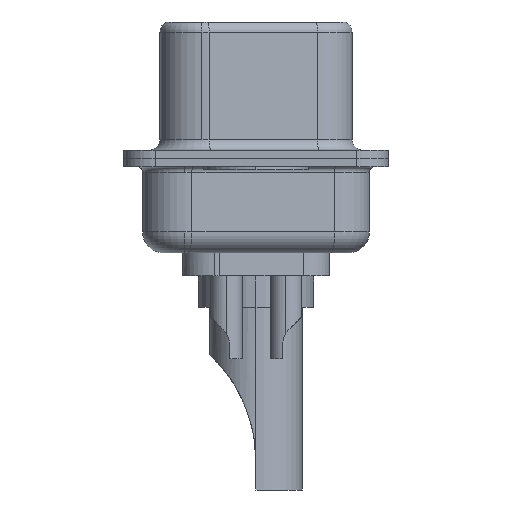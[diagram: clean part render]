
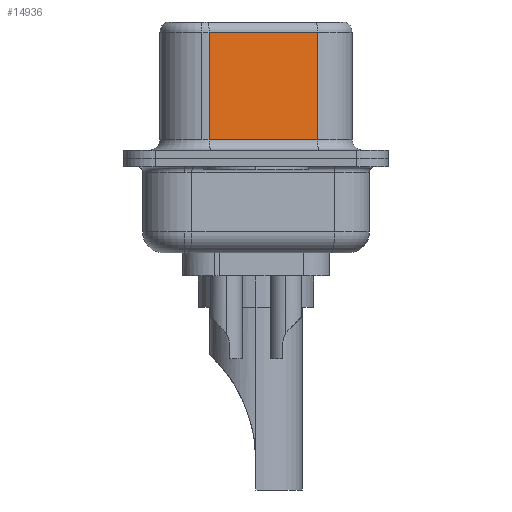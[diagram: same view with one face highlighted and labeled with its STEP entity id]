
A CAD part, left-side view. The second image highlights one B-rep face of the part: STEP entity #14936.
In plain terms, the highlighted planar face has unit normal (-0.985, -0.174, 0).
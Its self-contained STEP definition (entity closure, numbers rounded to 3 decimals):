
#769 = ORIENTED_EDGE ( 'NONE', *, *, #3355, .T. ) ;
#988 = DIRECTION ( 'NONE',  ( 0., 0., -1. ) ) ;
#1220 = VECTOR ( 'NONE', #13043, 1000. ) ;
#1666 = EDGE_CURVE ( 'NONE', #3581, #12307, #10937, .T. ) ;
#2328 = VECTOR ( 'NONE', #5864, 1000. ) ;
#3355 = EDGE_CURVE ( 'NONE', #6122, #3581, #7586, .T. ) ;
#3581 = VERTEX_POINT ( 'NONE', #12643 ) ;
#3767 = AXIS2_PLACEMENT_3D ( 'NONE', #15547, #12094, #4755 ) ;
#4089 = DIRECTION ( 'NONE',  ( 0., 0., -1. ) ) ;
#4755 = DIRECTION ( 'NONE',  ( -0.174, 0.985, 0. ) ) ;
#5244 = EDGE_LOOP ( 'NONE', ( #8255, #769, #15324, #13079 ) ) ;
#5864 = DIRECTION ( 'NONE',  ( 0.174, -0.985, 0. ) ) ;
#6122 = VERTEX_POINT ( 'NONE', #8403 ) ;
#6999 = FACE_OUTER_BOUND ( 'NONE', #5244, .T. ) ;
#7586 = LINE ( 'NONE', #11459, #1220 ) ;
#8171 = CARTESIAN_POINT ( 'NONE',  ( 4.565, -2.927, 6.52 ) ) ;
#8255 = ORIENTED_EDGE ( 'NONE', *, *, #9548, .F. ) ;
#8403 = CARTESIAN_POINT ( 'NONE',  ( 4.565, -2.927, 6.02 ) ) ;
#8763 = CARTESIAN_POINT ( 'NONE',  ( 3.655, 2.233, 6.52 ) ) ;
#9102 = VECTOR ( 'NONE', #988, 1000. ) ;
#9497 = LINE ( 'NONE', #8171, #9102 ) ;
#9548 = EDGE_CURVE ( 'NONE', #6122, #14612, #9497, .T. ) ;
#9572 = EDGE_CURVE ( 'NONE', #12307, #14612, #15115, .T. ) ;
#9593 = PLANE ( 'NONE',  #3767 ) ;
#10266 = CARTESIAN_POINT ( 'NONE',  ( 4.565, -2.927, 0.9 ) ) ;
#10937 = LINE ( 'NONE', #8763, #13698 ) ;
#11459 = CARTESIAN_POINT ( 'NONE',  ( 4.565, -2.927, 6.02 ) ) ;
#11978 = CARTESIAN_POINT ( 'NONE',  ( 4.565, -2.927, 0.9 ) ) ;
#12094 = DIRECTION ( 'NONE',  ( 0.985, 0.174, 0. ) ) ;
#12307 = VERTEX_POINT ( 'NONE', #14799 ) ;
#12643 = CARTESIAN_POINT ( 'NONE',  ( 3.655, 2.233, 6.02 ) ) ;
#13043 = DIRECTION ( 'NONE',  ( -0.174, 0.985, 0. ) ) ;
#13079 = ORIENTED_EDGE ( 'NONE', *, *, #9572, .T. ) ;
#13698 = VECTOR ( 'NONE', #4089, 1000. ) ;
#14612 = VERTEX_POINT ( 'NONE', #10266 ) ;
#14799 = CARTESIAN_POINT ( 'NONE',  ( 3.655, 2.233, 0.9 ) ) ;
#14936 = ADVANCED_FACE ( 'NONE', ( #6999 ), #9593, .F. ) ;
#15115 = LINE ( 'NONE', #11978, #2328 ) ;
#15324 = ORIENTED_EDGE ( 'NONE', *, *, #1666, .T. ) ;
#15547 = CARTESIAN_POINT ( 'NONE',  ( 4.565, -2.927, 6.52 ) ) ;
